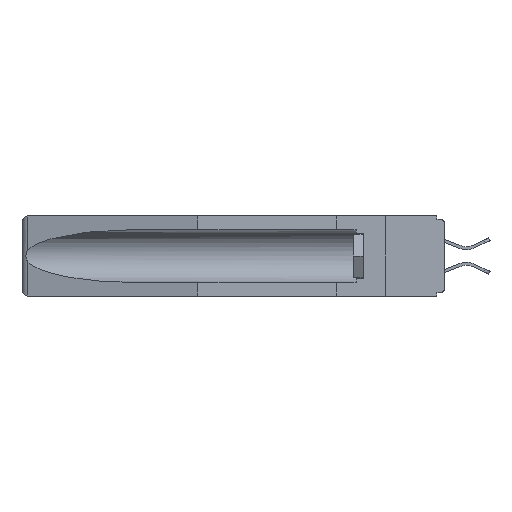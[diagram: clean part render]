
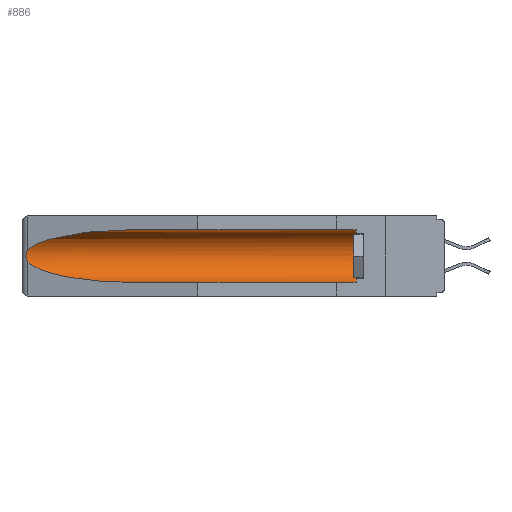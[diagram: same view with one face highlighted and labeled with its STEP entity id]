
A CAD part, left-side view. The second image highlights one B-rep face of the part: STEP entity #886.
In plain terms, the highlighted cylindrical face has radius 2.857 mm (diameter 5.715 mm), a partial arc.
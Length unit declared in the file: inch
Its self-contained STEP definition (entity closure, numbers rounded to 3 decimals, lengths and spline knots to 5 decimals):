
#886 = ADVANCED_FACE ( 'NONE', ( #14730 ), #18214, .F. ) ;
#903 = CARTESIAN_POINT ( 'NONE',  ( 0.21114, 1.30732, -0.284 ) ) ;
#1097 = ORIENTED_EDGE ( 'NONE', *, *, #6326, .T. ) ;
#1457 = CARTESIAN_POINT ( 'NONE',  ( 0.26655, 1.53094, -0.18657 ) ) ;
#2373 = CARTESIAN_POINT ( 'NONE',  ( 0.26537, 1.52718, -0.14972 ) ) ;
#2573 = CIRCLE ( 'NONE', #10158, 0.1125 ) ;
#3009 = CARTESIAN_POINT ( 'NONE',  ( 0.26654, 1.53092, -0.15636 ) ) ;
#3299 = CARTESIAN_POINT ( 'NONE',  ( 0.2673, 1.53269, -0.17917 ) ) ;
#3818 = LINE ( 'NONE', #11645, #17498 ) ;
#3870 = EDGE_CURVE ( 'NONE', #21233, #6054, #10946, .T. ) ;
#3964 =( BOUNDED_CURVE ( )  B_SPLINE_CURVE ( 3, ( #19862, #14837, #903, #16341 ),
 .UNSPECIFIED., .F., .T. ) 
 B_SPLINE_CURVE_WITH_KNOTS ( ( 4, 4 ),
 ( 0.1948, 1.5708 ),
 .UNSPECIFIED. ) 
 CURVE ( )  GEOMETRIC_REPRESENTATION_ITEM ( )  RATIONAL_B_SPLINE_CURVE ( ( 1., 0.848, 0.848, 1. ) ) 
 REPRESENTATION_ITEM ( '' )  );
#4302 = EDGE_LOOP ( 'NONE', ( #5198, #4858, #1097, #13671, #21393, #9251 ) ) ;
#4842 = DIRECTION ( 'NONE',  ( 0., 1., 0. ) ) ;
#4858 = ORIENTED_EDGE ( 'NONE', *, *, #16238, .T. ) ;
#5008 = CARTESIAN_POINT ( 'NONE',  ( 0.2675, 1.53308, -0.16763 ) ) ;
#5027 = EDGE_CURVE ( 'NONE', #16034, #17565, #2573, .T. ) ;
#5136 = CARTESIAN_POINT ( 'NONE',  ( 0.155, -0.30754, -0.059 ) ) ;
#5198 = ORIENTED_EDGE ( 'NONE', *, *, #3870, .T. ) ;
#6054 = VERTEX_POINT ( 'NONE', #6666 ) ;
#6206 = CARTESIAN_POINT ( 'NONE',  ( 0.155, 0.126, -0.1715 ) ) ;
#6326 = EDGE_CURVE ( 'NONE', #14778, #14534, #3964, .T. ) ;
#6457 = CARTESIAN_POINT ( 'NONE',  ( 0.26537, 1.52718, -0.19328 ) ) ;
#6666 = CARTESIAN_POINT ( 'NONE',  ( 0.26537, 1.52718, -0.14972 ) ) ;
#6669 = CARTESIAN_POINT ( 'NONE',  ( 0.2675, 1.53308, -0.17534 ) ) ;
#7020 = CARTESIAN_POINT ( 'NONE',  ( 0.155, 1.07973, -0.059 ) ) ;
#7535 = CARTESIAN_POINT ( 'NONE',  ( 0.155, 1.07973, -0.059 ) ) ;
#7698 = CARTESIAN_POINT ( 'NONE',  ( 0.25451, 1.48313, -0.09465 ) ) ;
#9251 = ORIENTED_EDGE ( 'NONE', *, *, #20888, .T. ) ;
#10158 = AXIS2_PLACEMENT_3D ( 'NONE', #6206, #14617, #11272 ) ;
#10803 = CARTESIAN_POINT ( 'NONE',  ( 0.21114, 1.30732, -0.059 ) ) ;
#10946 =( BOUNDED_CURVE ( )  B_SPLINE_CURVE ( 3, ( #7535, #10803, #7698, #2373 ),
 .UNSPECIFIED., .F., .T. ) 
 B_SPLINE_CURVE_WITH_KNOTS ( ( 4, 4 ),
 ( 4.71239, 6.08839 ),
 .UNSPECIFIED. ) 
 CURVE ( )  GEOMETRIC_REPRESENTATION_ITEM ( )  RATIONAL_B_SPLINE_CURVE ( ( 1., 0.848, 0.848, 1. ) ) 
 REPRESENTATION_ITEM ( '' )  );
#11272 = DIRECTION ( 'NONE',  ( 0., 0., 1. ) ) ;
#11645 = CARTESIAN_POINT ( 'NONE',  ( 0.155, -0.30754, -0.284 ) ) ;
#12747 = CARTESIAN_POINT ( 'NONE',  ( 0.155, -0.30754, -0.1715 ) ) ;
#13570 = DIRECTION ( 'NONE',  ( 0., 1., 0. ) ) ;
#13671 = ORIENTED_EDGE ( 'NONE', *, *, #16877, .F. ) ;
#14534 = VERTEX_POINT ( 'NONE', #14781 ) ;
#14617 = DIRECTION ( 'NONE',  ( 0., -1., 0. ) ) ;
#14730 = FACE_OUTER_BOUND ( 'NONE', #4302, .T. ) ;
#14778 = VERTEX_POINT ( 'NONE', #16741 ) ;
#14781 = CARTESIAN_POINT ( 'NONE',  ( 0.155, 1.07973, -0.284 ) ) ;
#14837 = CARTESIAN_POINT ( 'NONE',  ( 0.25451, 1.48313, -0.24835 ) ) ;
#15015 = CARTESIAN_POINT ( 'NONE',  ( 0.26597, 1.52961, -0.15275 ) ) ;
#15224 = VECTOR ( 'NONE', #13570, 39.37008 ) ;
#16034 = VERTEX_POINT ( 'NONE', #17949 ) ;
#16238 = EDGE_CURVE ( 'NONE', #6054, #14778, #21303, .T. ) ;
#16341 = CARTESIAN_POINT ( 'NONE',  ( 0.155, 1.07973, -0.284 ) ) ;
#16369 = CARTESIAN_POINT ( 'NONE',  ( 0.155, 0.126, -0.059 ) ) ;
#16741 = CARTESIAN_POINT ( 'NONE',  ( 0.26537, 1.52718, -0.19328 ) ) ;
#16819 = CARTESIAN_POINT ( 'NONE',  ( 0.2673, 1.5327, -0.16383 ) ) ;
#16877 = EDGE_CURVE ( 'NONE', #16034, #14534, #3818, .T. ) ;
#17498 = VECTOR ( 'NONE', #4842, 39.37008 ) ;
#17565 = VERTEX_POINT ( 'NONE', #16369 ) ;
#17887 = DIRECTION ( 'NONE',  ( 0., 1., 0. ) ) ;
#17949 = CARTESIAN_POINT ( 'NONE',  ( 0.155, 0.126, -0.284 ) ) ;
#17965 = DIRECTION ( 'NONE',  ( 0., 0., 1. ) ) ;
#18214 = CYLINDRICAL_SURFACE ( 'NONE', #18327, 0.1125 ) ;
#18327 = AXIS2_PLACEMENT_3D ( 'NONE', #12747, #17887, #17965 ) ;
#18705 = CARTESIAN_POINT ( 'NONE',  ( 0.26537, 1.52718, -0.14972 ) ) ;
#18712 = LINE ( 'NONE', #5136, #15224 ) ;
#19862 = CARTESIAN_POINT ( 'NONE',  ( 0.26537, 1.52718, -0.19328 ) ) ;
#20411 = CARTESIAN_POINT ( 'NONE',  ( 0.26597, 1.5296, -0.19026 ) ) ;
#20888 = EDGE_CURVE ( 'NONE', #17565, #21233, #18712, .T. ) ;
#21233 = VERTEX_POINT ( 'NONE', #7020 ) ;
#21303 = B_SPLINE_CURVE_WITH_KNOTS ( 'NONE', 3,
 ( #18705, #15015, #3009, #16819, #5008, #6669, #3299, #1457, #20411, #6457 ),
 .UNSPECIFIED., .F., .F.,
 ( 4, 2, 2, 2, 4 ),
 ( 0., 0.00029, 0.00058, 0.00087, 0.00117 ),
 .UNSPECIFIED. ) ;
#21393 = ORIENTED_EDGE ( 'NONE', *, *, #5027, .T. ) ;
